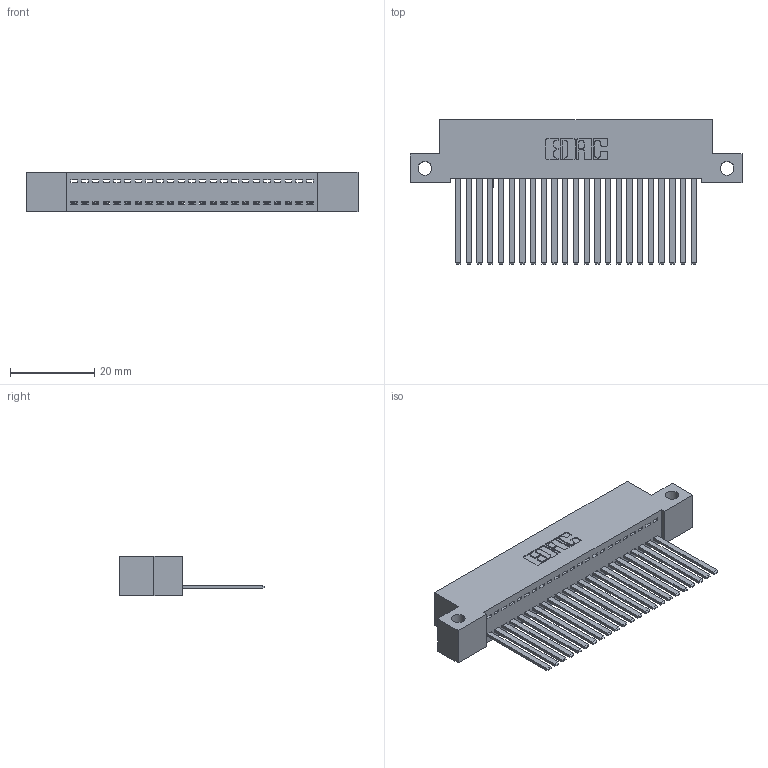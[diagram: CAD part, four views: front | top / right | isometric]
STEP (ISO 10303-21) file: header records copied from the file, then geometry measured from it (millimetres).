
FILE_DESCRIPTION (( 'STEP AP203' ), '1' );
FILE_NAME ('392-023-544-112.STEP', '2018-08-15T13:35:20', ( '' ), ( '' ), 'SwSTEP 2.0', 'SolidWorks 2016', '' );
FILE_SCHEMA (( 'CONFIG_CONTROL_DESIGN' ));
Length unit declared in the file: inch
Products named in the file (3): 342 Part_Side Mount; 345-292-001_345-293-144; 392-023-544-112
Assembly tree (24 placements, depth 2):
  392-023-544-112
    342 Part_Side Mount
    345-292-001_345-293-144  x23
Bounding box: 78.74 x 34.3 x 9.4 mm (x, y, z)
Volume: 7026.4 mm3; surface area: 10558.2 mm2
Topology: 24 solids, 24 shells, 1306 faces, 3933 edges, 2590 vertices
Faces by surface type: plane 940, cylinder 366
Entity records: 16205 total; most frequent: CARTESIAN_POINT 2803, ORIENTED_EDGE 2762, DIRECTION 2399, EDGE_CURVE 1381, VECTOR 1257, LINE 1257, VERTEX_POINT 918, AXIS2_PLACEMENT_3D 571
